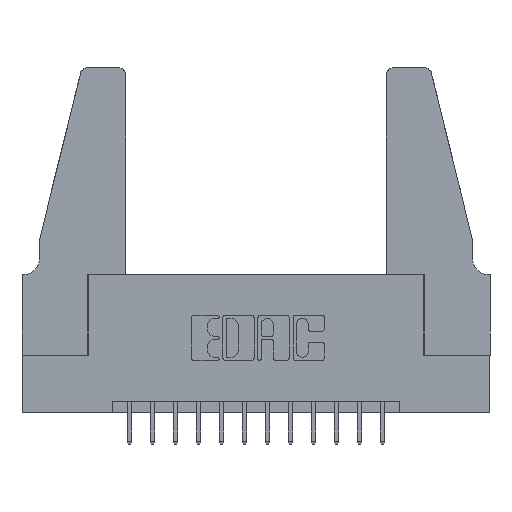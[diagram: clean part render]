
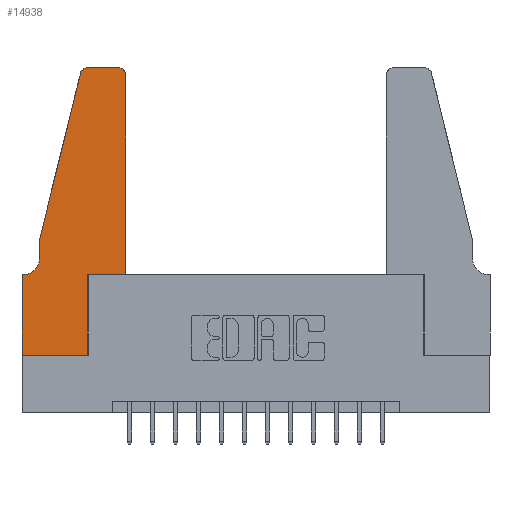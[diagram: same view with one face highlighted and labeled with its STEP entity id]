
A CAD part, top view. The second image highlights one B-rep face of the part: STEP entity #14938.
In plain terms, the highlighted planar face has unit normal (0, 0, 1).
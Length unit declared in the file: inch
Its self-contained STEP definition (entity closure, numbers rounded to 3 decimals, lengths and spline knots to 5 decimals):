
#56 = CARTESIAN_POINT ( 'NONE',  ( 0.4505, 0.35, 0.37 ) ) ;
#220 = DIRECTION ( 'NONE',  ( 1., 0., 0. ) ) ;
#408 = VERTEX_POINT ( 'NONE', #12064 ) ;
#624 = VERTEX_POINT ( 'NONE', #10010 ) ;
#865 = LINE ( 'NONE', #1898, #5007 ) ;
#909 = CIRCLE ( 'NONE', #7022, 0.03 ) ;
#916 = CARTESIAN_POINT ( 'NONE',  ( 0.0755, 0.5, 0.37 ) ) ;
#1102 = DIRECTION ( 'NONE',  ( 0., 0., -1. ) ) ;
#1181 = EDGE_CURVE ( 'NONE', #7889, #15129, #9895, .T. ) ;
#1310 = ORIENTED_EDGE ( 'NONE', *, *, #13479, .T. ) ;
#1728 = DIRECTION ( 'NONE',  ( 1., 0., 0. ) ) ;
#1784 = CARTESIAN_POINT ( 'NONE',  ( 0.25487, 1.22718, 0.37 ) ) ;
#1839 = ORIENTED_EDGE ( 'NONE', *, *, #8118, .T. ) ;
#1898 = CARTESIAN_POINT ( 'NONE',  ( 0.0755, 0.35, 0.37 ) ) ;
#1938 = VECTOR ( 'NONE', #2361, 39.37008 ) ;
#1979 = EDGE_CURVE ( 'NONE', #12037, #11353, #8866, .T. ) ;
#2255 = ORIENTED_EDGE ( 'NONE', *, *, #14770, .T. ) ;
#2344 = ORIENTED_EDGE ( 'NONE', *, *, #6888, .T. ) ;
#2361 = DIRECTION ( 'NONE',  ( 1., 0., 0. ) ) ;
#2362 = CARTESIAN_POINT ( 'NONE',  ( 0., 0., 0.37 ) ) ;
#2696 = ORIENTED_EDGE ( 'NONE', *, *, #13363, .T. ) ;
#2751 = VECTOR ( 'NONE', #7044, 39.37008 ) ;
#2775 = DIRECTION ( 'NONE',  ( 0., 1., 0. ) ) ;
#2945 = CARTESIAN_POINT ( 'NONE',  ( 0.2865, 0.35, 0.37 ) ) ;
#3080 = ORIENTED_EDGE ( 'NONE', *, *, #15620, .T. ) ;
#3269 = CARTESIAN_POINT ( 'NONE',  ( 0.4205, 1.25, 0.37 ) ) ;
#3349 = CARTESIAN_POINT ( 'NONE',  ( 0.0755, 0.42, 0.37 ) ) ;
#3613 = CARTESIAN_POINT ( 'NONE',  ( 0., 0., 0.37 ) ) ;
#4002 = VERTEX_POINT ( 'NONE', #1784 ) ;
#4129 = VERTEX_POINT ( 'NONE', #13325 ) ;
#4208 = LINE ( 'NONE', #2945, #4878 ) ;
#4528 = CARTESIAN_POINT ( 'NONE',  ( 0.4205, 1.22, 0.37 ) ) ;
#4604 = DIRECTION ( 'NONE',  ( 1., 0., 0. ) ) ;
#4650 = VECTOR ( 'NONE', #9418, 39.37008 ) ;
#4713 = ORIENTED_EDGE ( 'NONE', *, *, #1979, .T. ) ;
#4878 = VECTOR ( 'NONE', #2775, 39.37008 ) ;
#4932 = CARTESIAN_POINT ( 'NONE',  ( 0., 0.35, 0.37 ) ) ;
#5007 = VECTOR ( 'NONE', #6765, 39.37008 ) ;
#5207 = PLANE ( 'NONE',  #11619 ) ;
#5269 = VECTOR ( 'NONE', #220, 39.37008 ) ;
#5593 = VERTEX_POINT ( 'NONE', #14358 ) ;
#5819 = ORIENTED_EDGE ( 'NONE', *, *, #11266, .T. ) ;
#6023 = DIRECTION ( 'NONE',  ( 0., 1., 0. ) ) ;
#6128 = EDGE_CURVE ( 'NONE', #408, #14614, #9472, .T. ) ;
#6263 = ORIENTED_EDGE ( 'NONE', *, *, #6128, .T. ) ;
#6593 = FACE_OUTER_BOUND ( 'NONE', #8240, .T. ) ;
#6765 = DIRECTION ( 'NONE',  ( -1., 0., 0. ) ) ;
#6888 = EDGE_CURVE ( 'NONE', #15129, #4129, #4208, .T. ) ;
#7022 = AXIS2_PLACEMENT_3D ( 'NONE', #13347, #7324, #7976 ) ;
#7044 = DIRECTION ( 'NONE',  ( 0., -1., 0. ) ) ;
#7324 = DIRECTION ( 'NONE',  ( 0., 0., 1. ) ) ;
#7392 = DIRECTION ( 'NONE',  ( -1., 0., 0. ) ) ;
#7628 = VECTOR ( 'NONE', #15086, 39.37008 ) ;
#7889 = VERTEX_POINT ( 'NONE', #15185 ) ;
#7976 = DIRECTION ( 'NONE',  ( 1., 0., 0. ) ) ;
#8064 = CIRCLE ( 'NONE', #11092, 0.07 ) ;
#8118 = EDGE_CURVE ( 'NONE', #4002, #408, #11683, .T. ) ;
#8240 = EDGE_LOOP ( 'NONE', ( #4713, #5819, #1839, #6263, #11417, #14009, #3080, #9457, #2344, #1310, #2255, #2696 ) ) ;
#8290 = DIRECTION ( 'NONE',  ( 0., -1., 0. ) ) ;
#8866 = LINE ( 'NONE', #10212, #7628 ) ;
#9032 = DIRECTION ( 'NONE',  ( 0., 0., 1. ) ) ;
#9418 = DIRECTION ( 'NONE',  ( -0.239, -0.971, 0. ) ) ;
#9424 = CARTESIAN_POINT ( 'NONE',  ( 0.2865, 0., 0.37 ) ) ;
#9457 = ORIENTED_EDGE ( 'NONE', *, *, #1181, .T. ) ;
#9472 = LINE ( 'NONE', #14337, #15306 ) ;
#9680 = VERTEX_POINT ( 'NONE', #15600 ) ;
#9895 = LINE ( 'NONE', #2362, #5269 ) ;
#10010 = CARTESIAN_POINT ( 'NONE',  ( 0.0055, 0.35, 0.37 ) ) ;
#10212 = CARTESIAN_POINT ( 'NONE',  ( 0.2605, 1.25, 0.37 ) ) ;
#11004 = CARTESIAN_POINT ( 'NONE',  ( 0.284, 1.25, 0.37 ) ) ;
#11092 = AXIS2_PLACEMENT_3D ( 'NONE', #14696, #1102, #7392 ) ;
#11266 = EDGE_CURVE ( 'NONE', #11353, #4002, #909, .T. ) ;
#11353 = VERTEX_POINT ( 'NONE', #11004 ) ;
#11398 = CARTESIAN_POINT ( 'NONE',  ( 0., 0.35, 0.37 ) ) ;
#11417 = ORIENTED_EDGE ( 'NONE', *, *, #14787, .T. ) ;
#11619 = AXIS2_PLACEMENT_3D ( 'NONE', #11398, #9032, #1728 ) ;
#11683 = LINE ( 'NONE', #916, #4650 ) ;
#11830 = DIRECTION ( 'NONE',  ( 0., 0., 1. ) ) ;
#12037 = VERTEX_POINT ( 'NONE', #3269 ) ;
#12064 = CARTESIAN_POINT ( 'NONE',  ( 0.0755, 0.5, 0.37 ) ) ;
#12100 = CIRCLE ( 'NONE', #14888, 0.03 ) ;
#12154 = CARTESIAN_POINT ( 'NONE',  ( 0.4505, 0.35, 0.37 ) ) ;
#12188 = VERTEX_POINT ( 'NONE', #4932 ) ;
#13199 = LINE ( 'NONE', #12154, #14913 ) ;
#13325 = CARTESIAN_POINT ( 'NONE',  ( 0.2865, 0.35, 0.37 ) ) ;
#13347 = CARTESIAN_POINT ( 'NONE',  ( 0.284, 1.22, 0.37 ) ) ;
#13363 = EDGE_CURVE ( 'NONE', #9680, #12037, #12100, .T. ) ;
#13479 = EDGE_CURVE ( 'NONE', #4129, #5593, #14692, .T. ) ;
#14009 = ORIENTED_EDGE ( 'NONE', *, *, #14623, .T. ) ;
#14337 = CARTESIAN_POINT ( 'NONE',  ( 0.0755, 0.5, 0.37 ) ) ;
#14358 = CARTESIAN_POINT ( 'NONE',  ( 0.4505, 0.35, 0.37 ) ) ;
#14429 = LINE ( 'NONE', #3613, #2751 ) ;
#14614 = VERTEX_POINT ( 'NONE', #3349 ) ;
#14623 = EDGE_CURVE ( 'NONE', #624, #12188, #865, .T. ) ;
#14692 = LINE ( 'NONE', #56, #1938 ) ;
#14696 = CARTESIAN_POINT ( 'NONE',  ( 0.0055, 0.42, 0.37 ) ) ;
#14770 = EDGE_CURVE ( 'NONE', #5593, #9680, #13199, .T. ) ;
#14787 = EDGE_CURVE ( 'NONE', #14614, #624, #8064, .T. ) ;
#14888 = AXIS2_PLACEMENT_3D ( 'NONE', #4528, #11830, #4604 ) ;
#14913 = VECTOR ( 'NONE', #6023, 39.37008 ) ;
#14938 = ADVANCED_FACE ( 'NONE', ( #6593 ), #5207, .T. ) ;
#15086 = DIRECTION ( 'NONE',  ( -1., 0., 0. ) ) ;
#15129 = VERTEX_POINT ( 'NONE', #9424 ) ;
#15185 = CARTESIAN_POINT ( 'NONE',  ( 0., 0., 0.37 ) ) ;
#15306 = VECTOR ( 'NONE', #8290, 39.37008 ) ;
#15600 = CARTESIAN_POINT ( 'NONE',  ( 0.4505, 1.22, 0.37 ) ) ;
#15620 = EDGE_CURVE ( 'NONE', #12188, #7889, #14429, .T. ) ;
